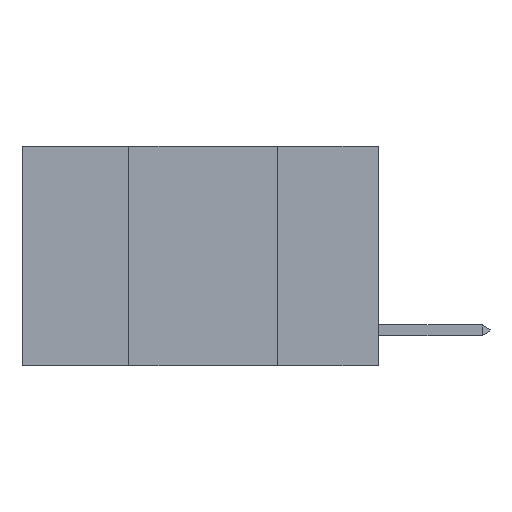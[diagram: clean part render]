
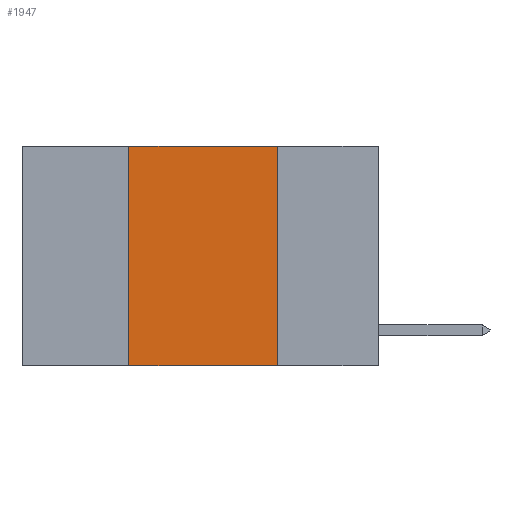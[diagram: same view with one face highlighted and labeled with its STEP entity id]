
A CAD part, left-side view. The second image highlights one B-rep face of the part: STEP entity #1947.
In plain terms, the highlighted planar face has unit normal (-1, 0, 0).
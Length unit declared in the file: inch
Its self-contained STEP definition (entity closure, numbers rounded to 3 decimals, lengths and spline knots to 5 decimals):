
#70 = CARTESIAN_POINT ( 'NONE',  ( 0., 0.17, 0. ) ) ;
#763 = CARTESIAN_POINT ( 'NONE',  ( 0., 0.6, 0. ) ) ;
#1947 = ADVANCED_FACE ( 'NONE', ( #16153 ), #14715, .F. ) ;
#4405 = EDGE_CURVE ( 'NONE', #17347, #17736, #16602, .T. ) ;
#5206 = CARTESIAN_POINT ( 'NONE',  ( 0., 0.6, 0. ) ) ;
#5374 = VERTEX_POINT ( 'NONE', #14461 ) ;
#5490 = DIRECTION ( 'NONE',  ( 0., -1., 0. ) ) ;
#5728 = CARTESIAN_POINT ( 'NONE',  ( 0., 0.42, 0. ) ) ;
#5764 = CARTESIAN_POINT ( 'NONE',  ( 0., 0.6, -0.37 ) ) ;
#5780 = VECTOR ( 'NONE', #5490, 39.37008 ) ;
#6230 = EDGE_CURVE ( 'NONE', #5374, #17736, #14922, .T. ) ;
#6355 = DIRECTION ( 'NONE',  ( 0., 0., -1. ) ) ;
#6799 = ORIENTED_EDGE ( 'NONE', *, *, #6230, .F. ) ;
#6844 = DIRECTION ( 'NONE',  ( 0., 0., 1. ) ) ;
#7390 = VECTOR ( 'NONE', #6844, 39.37008 ) ;
#7423 = DIRECTION ( 'NONE',  ( 0., -1., 0. ) ) ;
#8578 = LINE ( 'NONE', #763, #5780 ) ;
#9649 = DIRECTION ( 'NONE',  ( 0., 0., -1. ) ) ;
#9812 = LINE ( 'NONE', #16026, #7390 ) ;
#11042 = CARTESIAN_POINT ( 'NONE',  ( 0., 0.42, -0.37 ) ) ;
#11750 = ORIENTED_EDGE ( 'NONE', *, *, #4405, .T. ) ;
#12815 = CARTESIAN_POINT ( 'NONE',  ( 0., 0.17, -0.37 ) ) ;
#12848 = ORIENTED_EDGE ( 'NONE', *, *, #12882, .F. ) ;
#12882 = EDGE_CURVE ( 'NONE', #17347, #19873, #9812, .T. ) ;
#13800 = VECTOR ( 'NONE', #6355, 39.37008 ) ;
#14321 = DIRECTION ( 'NONE',  ( 1., 0., 0. ) ) ;
#14461 = CARTESIAN_POINT ( 'NONE',  ( 0., 0.17, 0. ) ) ;
#14715 = PLANE ( 'NONE',  #19072 ) ;
#14922 = LINE ( 'NONE', #70, #13800 ) ;
#15146 = EDGE_LOOP ( 'NONE', ( #6799, #20196, #12848, #11750 ) ) ;
#15794 = EDGE_CURVE ( 'NONE', #19873, #5374, #8578, .T. ) ;
#16026 = CARTESIAN_POINT ( 'NONE',  ( 0., 0.42, 0. ) ) ;
#16153 = FACE_OUTER_BOUND ( 'NONE', #15146, .T. ) ;
#16602 = LINE ( 'NONE', #5764, #17911 ) ;
#17347 = VERTEX_POINT ( 'NONE', #11042 ) ;
#17736 = VERTEX_POINT ( 'NONE', #12815 ) ;
#17911 = VECTOR ( 'NONE', #7423, 39.37008 ) ;
#19072 = AXIS2_PLACEMENT_3D ( 'NONE', #5206, #14321, #9649 ) ;
#19873 = VERTEX_POINT ( 'NONE', #5728 ) ;
#20196 = ORIENTED_EDGE ( 'NONE', *, *, #15794, .F. ) ;
